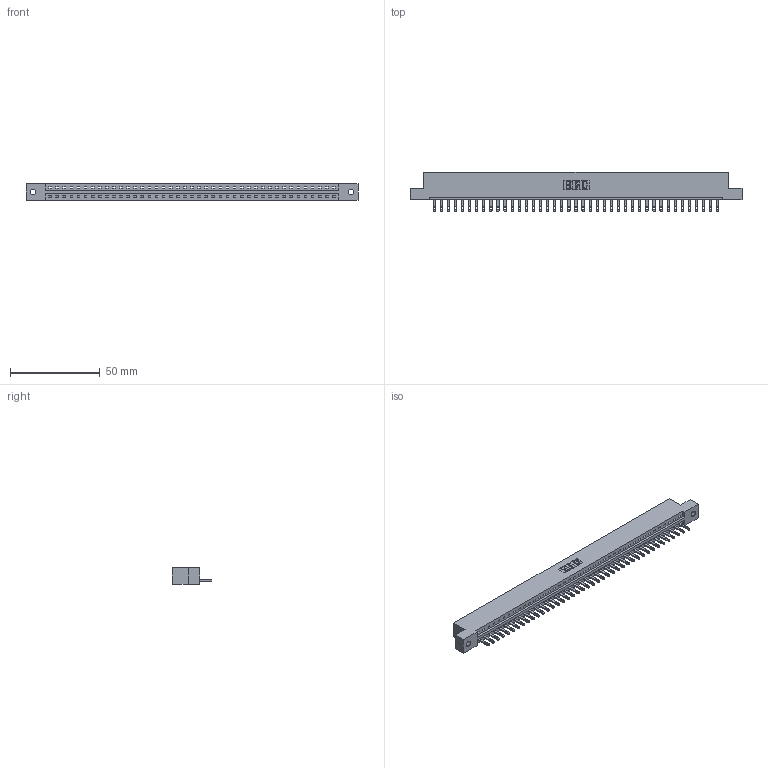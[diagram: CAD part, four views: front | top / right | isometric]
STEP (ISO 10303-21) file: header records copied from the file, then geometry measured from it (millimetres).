
FILE_DESCRIPTION (( 'STEP AP203' ), '1' );
FILE_NAME ('337-041-500-102.STEP', '2019-10-01T20:13:46', ( '' ), ( '' ), 'SwSTEP 2.0', 'SolidWorks 2016', '' );
FILE_SCHEMA (( 'CONFIG_CONTROL_DESIGN' ));
Length unit declared in the file: inch
Products named in the file (3): 345-292-001_345-293-100; 337 Part_Flush Mounting Lugs - 0.128 Dia; 337-041-500-102
Assembly tree (42 placements, depth 2):
  337-041-500-102
    337 Part_Flush Mounting Lugs - 0.128 Dia
    345-292-001_345-293-100  x41
Bounding box: 185.47 x 21.85 x 9.4 mm (x, y, z)
Volume: 19252.8 mm3; surface area: 19715.2 mm2
Topology: 42 solids, 42 shells, 2492 faces, 7691 edges, 5126 vertices
Faces by surface type: plane 1710, cylinder 782
Entity records: 30539 total; most frequent: CARTESIAN_POINT 5325, ORIENTED_EDGE 5302, DIRECTION 4485, EDGE_CURVE 2651, VECTOR 2519, LINE 2519, VERTEX_POINT 1766, AXIS2_PLACEMENT_3D 983
